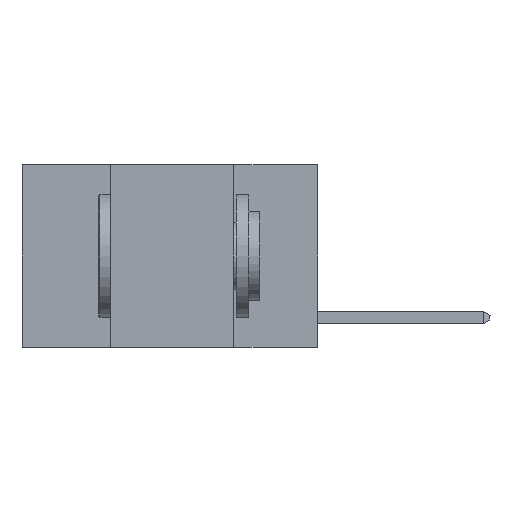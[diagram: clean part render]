
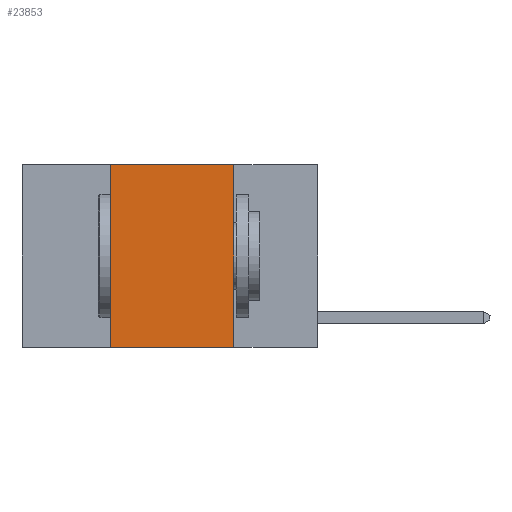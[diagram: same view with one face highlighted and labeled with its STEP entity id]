
A CAD part, left-side view. The second image highlights one B-rep face of the part: STEP entity #23853.
In plain terms, the highlighted planar face has unit normal (-1, 0, 0).
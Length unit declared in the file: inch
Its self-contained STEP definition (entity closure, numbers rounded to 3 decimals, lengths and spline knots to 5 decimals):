
#194 = CARTESIAN_POINT ( 'NONE',  ( 0., 0.17, 0. ) ) ;
#448 = DIRECTION ( 'NONE',  ( 0., 0., -1. ) ) ;
#1394 = VERTEX_POINT ( 'NONE', #17740 ) ;
#2279 = EDGE_CURVE ( 'NONE', #24682, #11175, #14828, .T. ) ;
#2418 = DIRECTION ( 'NONE',  ( 0., 0., -1. ) ) ;
#4117 = CARTESIAN_POINT ( 'NONE',  ( 0., 0.42, 0. ) ) ;
#5864 = CARTESIAN_POINT ( 'NONE',  ( 0., 0.6, -0.37 ) ) ;
#6260 = LINE ( 'NONE', #5864, #16610 ) ;
#6441 = VECTOR ( 'NONE', #2418, 39.37008 ) ;
#7050 = EDGE_CURVE ( 'NONE', #27642, #1394, #6260, .T. ) ;
#8086 = DIRECTION ( 'NONE',  ( 0., -1., 0. ) ) ;
#8135 = VECTOR ( 'NONE', #14840, 39.37008 ) ;
#11100 = ORIENTED_EDGE ( 'NONE', *, *, #2279, .F. ) ;
#11175 = VERTEX_POINT ( 'NONE', #26776 ) ;
#11440 = CARTESIAN_POINT ( 'NONE',  ( 0., 0.6, 0. ) ) ;
#11639 = LINE ( 'NONE', #194, #6441 ) ;
#11795 = ORIENTED_EDGE ( 'NONE', *, *, #7050, .T. ) ;
#12423 = EDGE_CURVE ( 'NONE', #11175, #1394, #11639, .T. ) ;
#12966 = EDGE_CURVE ( 'NONE', #27642, #24682, #19861, .T. ) ;
#13610 = DIRECTION ( 'NONE',  ( 1., 0., 0. ) ) ;
#14828 = LINE ( 'NONE', #16329, #25751 ) ;
#14840 = DIRECTION ( 'NONE',  ( 0., 0., 1. ) ) ;
#15244 = EDGE_LOOP ( 'NONE', ( #27793, #11100, #22736, #11795 ) ) ;
#16329 = CARTESIAN_POINT ( 'NONE',  ( 0., 0.6, 0. ) ) ;
#16610 = VECTOR ( 'NONE', #8086, 39.37008 ) ;
#16980 = CARTESIAN_POINT ( 'NONE',  ( 0., 0.42, 0. ) ) ;
#17740 = CARTESIAN_POINT ( 'NONE',  ( 0., 0.17, -0.37 ) ) ;
#19861 = LINE ( 'NONE', #16980, #8135 ) ;
#21458 = CARTESIAN_POINT ( 'NONE',  ( 0., 0.42, -0.37 ) ) ;
#22736 = ORIENTED_EDGE ( 'NONE', *, *, #12966, .F. ) ;
#23499 = FACE_OUTER_BOUND ( 'NONE', #15244, .T. ) ;
#23853 = ADVANCED_FACE ( 'NONE', ( #23499 ), #26667, .F. ) ;
#24682 = VERTEX_POINT ( 'NONE', #4117 ) ;
#24988 = AXIS2_PLACEMENT_3D ( 'NONE', #11440, #13610, #448 ) ;
#25751 = VECTOR ( 'NONE', #27142, 39.37008 ) ;
#26667 = PLANE ( 'NONE',  #24988 ) ;
#26776 = CARTESIAN_POINT ( 'NONE',  ( 0., 0.17, 0. ) ) ;
#27142 = DIRECTION ( 'NONE',  ( 0., -1., 0. ) ) ;
#27642 = VERTEX_POINT ( 'NONE', #21458 ) ;
#27793 = ORIENTED_EDGE ( 'NONE', *, *, #12423, .F. ) ;
